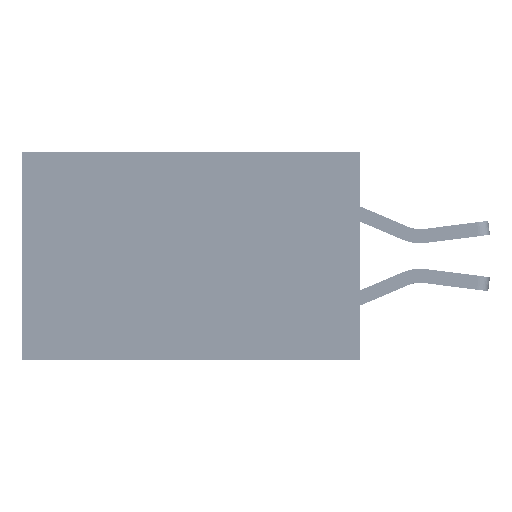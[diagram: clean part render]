
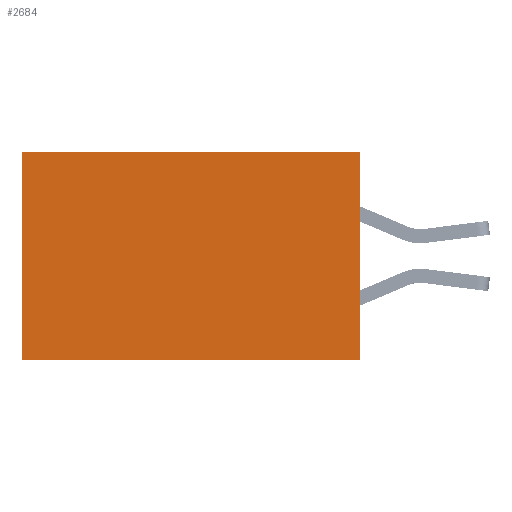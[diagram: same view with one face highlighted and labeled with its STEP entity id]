
A CAD part, left-side view. The second image highlights one B-rep face of the part: STEP entity #2684.
In plain terms, the highlighted planar face has unit normal (-1, 0, 0).
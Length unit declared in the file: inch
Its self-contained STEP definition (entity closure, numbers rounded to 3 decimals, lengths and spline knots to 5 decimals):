
#2684 = ADVANCED_FACE ( 'NONE', ( #14559 ), #6699, .F. ) ;
#5989 = LINE ( 'NONE', #16675, #32345 ) ;
#6699 = PLANE ( 'NONE',  #21844 ) ;
#7476 = VERTEX_POINT ( 'NONE', #20080 ) ;
#8829 = VECTOR ( 'NONE', #15636, 39.37008 ) ;
#11118 = DIRECTION ( 'NONE',  ( 0., 1., 0. ) ) ;
#12390 = ORIENTED_EDGE ( 'NONE', *, *, #24964, .F. ) ;
#14559 = FACE_OUTER_BOUND ( 'NONE', #23924, .T. ) ;
#14710 = ORIENTED_EDGE ( 'NONE', *, *, #30486, .T. ) ;
#15636 = DIRECTION ( 'NONE',  ( 0., 1., 0. ) ) ;
#16675 = CARTESIAN_POINT ( 'NONE',  ( 0.2875, 0., -0.37 ) ) ;
#19529 = VECTOR ( 'NONE', #30557, 39.37008 ) ;
#19768 = ORIENTED_EDGE ( 'NONE', *, *, #32627, .F. ) ;
#20080 = CARTESIAN_POINT ( 'NONE',  ( 0.2875, 0.6, 0. ) ) ;
#20353 = VERTEX_POINT ( 'NONE', #21370 ) ;
#20831 = DIRECTION ( 'NONE',  ( 1., 0., 0. ) ) ;
#21370 = CARTESIAN_POINT ( 'NONE',  ( 0.2875, 0., 0. ) ) ;
#21526 = CARTESIAN_POINT ( 'NONE',  ( 0.2875, 0.6, -0.37 ) ) ;
#21700 = CARTESIAN_POINT ( 'NONE',  ( 0.2875, 0.6, 0. ) ) ;
#21844 = AXIS2_PLACEMENT_3D ( 'NONE', #28700, #20831, #26710 ) ;
#22009 = VECTOR ( 'NONE', #24451, 39.37008 ) ;
#22773 = VERTEX_POINT ( 'NONE', #29059 ) ;
#23924 = EDGE_LOOP ( 'NONE', ( #27122, #19768, #12390, #14710 ) ) ;
#24451 = DIRECTION ( 'NONE',  ( 0., 0., -1. ) ) ;
#24964 = EDGE_CURVE ( 'NONE', #20353, #22773, #30687, .T. ) ;
#26710 = DIRECTION ( 'NONE',  ( 0., 0., -1. ) ) ;
#27122 = ORIENTED_EDGE ( 'NONE', *, *, #35894, .T. ) ;
#28700 = CARTESIAN_POINT ( 'NONE',  ( 0.2875, 0., 0. ) ) ;
#29059 = CARTESIAN_POINT ( 'NONE',  ( 0.2875, 0., -0.37 ) ) ;
#29388 = LINE ( 'NONE', #33088, #8829 ) ;
#30486 = EDGE_CURVE ( 'NONE', #20353, #7476, #29388, .T. ) ;
#30557 = DIRECTION ( 'NONE',  ( 0., 0., -1. ) ) ;
#30687 = LINE ( 'NONE', #36421, #19529 ) ;
#32345 = VECTOR ( 'NONE', #11118, 39.37008 ) ;
#32627 = EDGE_CURVE ( 'NONE', #22773, #34466, #5989, .T. ) ;
#33088 = CARTESIAN_POINT ( 'NONE',  ( 0.2875, 0., 0. ) ) ;
#34030 = LINE ( 'NONE', #21700, #22009 ) ;
#34466 = VERTEX_POINT ( 'NONE', #21526 ) ;
#35894 = EDGE_CURVE ( 'NONE', #7476, #34466, #34030, .T. ) ;
#36421 = CARTESIAN_POINT ( 'NONE',  ( 0.2875, 0., 0. ) ) ;
